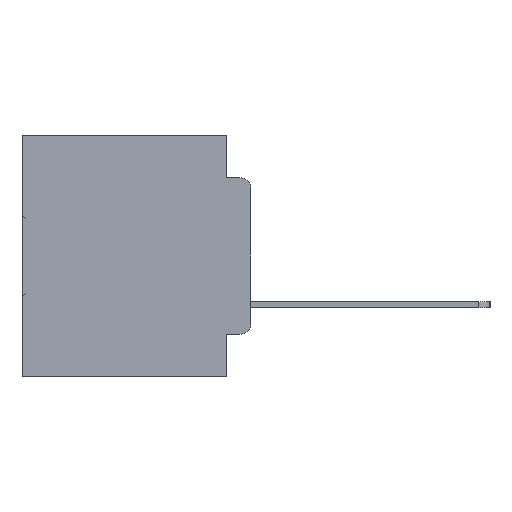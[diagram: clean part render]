
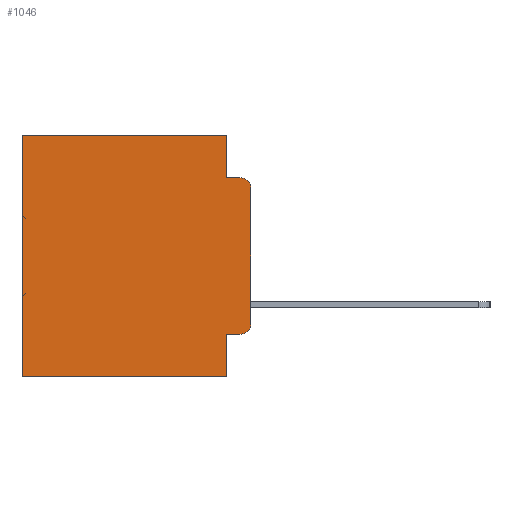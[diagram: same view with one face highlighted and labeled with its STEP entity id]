
A CAD part, left-side view. The second image highlights one B-rep face of the part: STEP entity #1046.
In plain terms, the highlighted planar face has unit normal (-1, 0, 0).
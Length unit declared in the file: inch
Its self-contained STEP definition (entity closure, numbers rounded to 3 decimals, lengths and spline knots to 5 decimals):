
#7 = ORIENTED_EDGE ( 'NONE', *, *, #6606, .T. ) ;
#1046 = ADVANCED_FACE ( 'NONE', ( #17007 ), #32919, .F. ) ;
#1188 = DIRECTION ( 'NONE',  ( 0., 0., -1. ) ) ;
#1389 = CARTESIAN_POINT ( 'NONE',  ( 0.298, 0.051, -0.0885 ) ) ;
#1459 = EDGE_LOOP ( 'NONE', ( #22187, #8716, #4478, #12421, #5439, #13351, #21767, #29298, #7, #10144 ) ) ;
#2186 = CARTESIAN_POINT ( 'NONE',  ( 0.298, 0.473, 0. ) ) ;
#3170 = EDGE_CURVE ( 'NONE', #9310, #4926, #35916, .T. ) ;
#3719 = CARTESIAN_POINT ( 'NONE',  ( 0.298, 0., 0. ) ) ;
#3801 = EDGE_CURVE ( 'NONE', #24891, #9053, #29232, .T. ) ;
#4478 = ORIENTED_EDGE ( 'NONE', *, *, #23325, .F. ) ;
#4813 = AXIS2_PLACEMENT_3D ( 'NONE', #27524, #13738, #1188 ) ;
#4926 = VERTEX_POINT ( 'NONE', #19054 ) ;
#5336 = EDGE_CURVE ( 'NONE', #36513, #9310, #36146, .T. ) ;
#5339 = EDGE_CURVE ( 'NONE', #24891, #35664, #14929, .T. ) ;
#5353 = VECTOR ( 'NONE', #25666, 39.37008 ) ;
#5439 = ORIENTED_EDGE ( 'NONE', *, *, #5339, .T. ) ;
#5473 = VERTEX_POINT ( 'NONE', #21811 ) ;
#6214 = DIRECTION ( 'NONE',  ( 0., 0., -1. ) ) ;
#6606 = EDGE_CURVE ( 'NONE', #36513, #32091, #26537, .T. ) ;
#6811 = DIRECTION ( 'NONE',  ( 0., 1., 0. ) ) ;
#7334 = EDGE_CURVE ( 'NONE', #32091, #5473, #15463, .T. ) ;
#8716 = ORIENTED_EDGE ( 'NONE', *, *, #25232, .T. ) ;
#9053 = VERTEX_POINT ( 'NONE', #17117 ) ;
#9116 = CARTESIAN_POINT ( 'NONE',  ( 0.298, 0.02, -0.1085 ) ) ;
#9310 = VERTEX_POINT ( 'NONE', #26524 ) ;
#10144 = ORIENTED_EDGE ( 'NONE', *, *, #7334, .T. ) ;
#10627 = DIRECTION ( 'NONE',  ( 0., 1., 0. ) ) ;
#10633 = CARTESIAN_POINT ( 'NONE',  ( 0.298, 0.051, -0.4115 ) ) ;
#12115 = DIRECTION ( 'NONE',  ( 0., 0., -1. ) ) ;
#12421 = ORIENTED_EDGE ( 'NONE', *, *, #3801, .F. ) ;
#12759 = VERTEX_POINT ( 'NONE', #17039 ) ;
#13265 = DIRECTION ( 'NONE',  ( 0., 0., -1. ) ) ;
#13351 = ORIENTED_EDGE ( 'NONE', *, *, #31658, .T. ) ;
#13563 = DIRECTION ( 'NONE',  ( 0., -1., 0. ) ) ;
#13738 = DIRECTION ( 'NONE',  ( 1., 0., 0. ) ) ;
#14019 = CARTESIAN_POINT ( 'NONE',  ( 0.298, 0.02, -0.4115 ) ) ;
#14057 = VECTOR ( 'NONE', #15538, 39.37008 ) ;
#14144 = DIRECTION ( 'NONE',  ( -1., 0., 0. ) ) ;
#14929 = LINE ( 'NONE', #3719, #35333 ) ;
#14949 = LINE ( 'NONE', #23504, #35350 ) ;
#15062 = VECTOR ( 'NONE', #10627, 39.37008 ) ;
#15463 = CIRCLE ( 'NONE', #21778, 0.02 ) ;
#15538 = DIRECTION ( 'NONE',  ( 0., 0., -1. ) ) ;
#16357 = LINE ( 'NONE', #32762, #36585 ) ;
#16438 = DIRECTION ( 'NONE',  ( 0., -1., 0. ) ) ;
#17007 = FACE_OUTER_BOUND ( 'NONE', #1459, .T. ) ;
#17039 = CARTESIAN_POINT ( 'NONE',  ( 0.298, 0.02, -0.0885 ) ) ;
#17117 = CARTESIAN_POINT ( 'NONE',  ( 0.298, 0.051, -0.0885 ) ) ;
#18121 = VECTOR ( 'NONE', #13563, 39.37008 ) ;
#18395 = VERTEX_POINT ( 'NONE', #33103 ) ;
#19054 = CARTESIAN_POINT ( 'NONE',  ( 0.298, 0.473, -0.5 ) ) ;
#21419 = EDGE_CURVE ( 'NONE', #18395, #5473, #16357, .T. ) ;
#21767 = ORIENTED_EDGE ( 'NONE', *, *, #3170, .F. ) ;
#21778 = AXIS2_PLACEMENT_3D ( 'NONE', #30996, #14144, #33637 ) ;
#21811 = CARTESIAN_POINT ( 'NONE',  ( 0.298, 0., -0.3915 ) ) ;
#22086 = CARTESIAN_POINT ( 'NONE',  ( 0.298, 0., -0.5 ) ) ;
#22187 = ORIENTED_EDGE ( 'NONE', *, *, #21419, .F. ) ;
#22815 = AXIS2_PLACEMENT_3D ( 'NONE', #9116, #29113, #12115 ) ;
#23251 = CARTESIAN_POINT ( 'NONE',  ( 0.298, 0.051, -0.4115 ) ) ;
#23325 = EDGE_CURVE ( 'NONE', #9053, #12759, #36472, .T. ) ;
#23504 = CARTESIAN_POINT ( 'NONE',  ( 0.298, 0.473, 0. ) ) ;
#24595 = VECTOR ( 'NONE', #16438, 39.37008 ) ;
#24891 = VERTEX_POINT ( 'NONE', #30109 ) ;
#25232 = EDGE_CURVE ( 'NONE', #18395, #12759, #33645, .T. ) ;
#25666 = DIRECTION ( 'NONE',  ( 0., 0., -1. ) ) ;
#26524 = CARTESIAN_POINT ( 'NONE',  ( 0.298, 0.051, -0.5 ) ) ;
#26537 = LINE ( 'NONE', #10633, #18121 ) ;
#27524 = CARTESIAN_POINT ( 'NONE',  ( 0.298, 0., 0. ) ) ;
#28517 = CARTESIAN_POINT ( 'NONE',  ( 0.298, 0.051, 0. ) ) ;
#29113 = DIRECTION ( 'NONE',  ( -1., 0., 0. ) ) ;
#29232 = LINE ( 'NONE', #28517, #5353 ) ;
#29298 = ORIENTED_EDGE ( 'NONE', *, *, #5336, .F. ) ;
#30109 = CARTESIAN_POINT ( 'NONE',  ( 0.298, 0.051, 0. ) ) ;
#30996 = CARTESIAN_POINT ( 'NONE',  ( 0.298, 0.02, -0.3915 ) ) ;
#31658 = EDGE_CURVE ( 'NONE', #35664, #4926, #14949, .T. ) ;
#32091 = VERTEX_POINT ( 'NONE', #14019 ) ;
#32318 = CARTESIAN_POINT ( 'NONE',  ( 0.298, 0.051, 0. ) ) ;
#32762 = CARTESIAN_POINT ( 'NONE',  ( 0.298, 0., 0. ) ) ;
#32919 = PLANE ( 'NONE',  #4813 ) ;
#33103 = CARTESIAN_POINT ( 'NONE',  ( 0.298, 0., -0.1085 ) ) ;
#33637 = DIRECTION ( 'NONE',  ( 0., 0., -1. ) ) ;
#33645 = CIRCLE ( 'NONE', #22815, 0.02 ) ;
#35333 = VECTOR ( 'NONE', #6811, 39.37008 ) ;
#35350 = VECTOR ( 'NONE', #6214, 39.37008 ) ;
#35664 = VERTEX_POINT ( 'NONE', #2186 ) ;
#35916 = LINE ( 'NONE', #22086, #15062 ) ;
#36146 = LINE ( 'NONE', #32318, #14057 ) ;
#36472 = LINE ( 'NONE', #1389, #24595 ) ;
#36513 = VERTEX_POINT ( 'NONE', #23251 ) ;
#36585 = VECTOR ( 'NONE', #13265, 39.37008 ) ;
